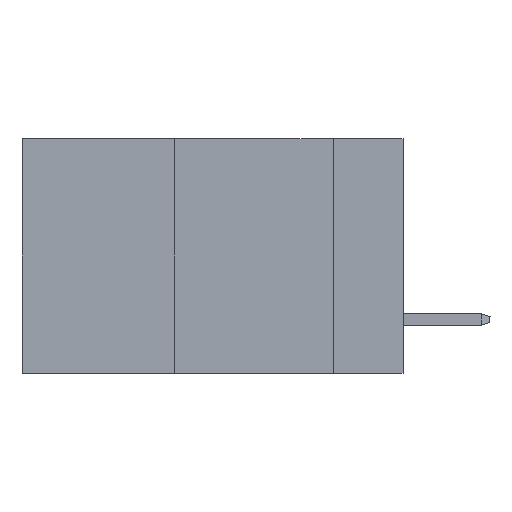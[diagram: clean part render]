
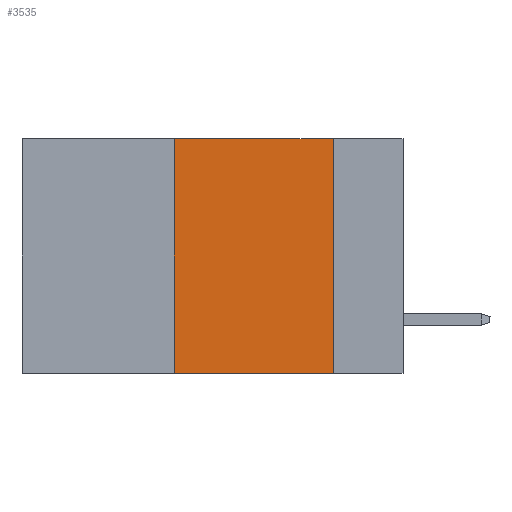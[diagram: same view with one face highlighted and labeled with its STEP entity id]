
A CAD part, left-side view. The second image highlights one B-rep face of the part: STEP entity #3535.
In plain terms, the highlighted planar face has unit normal (-1, 0, 0).
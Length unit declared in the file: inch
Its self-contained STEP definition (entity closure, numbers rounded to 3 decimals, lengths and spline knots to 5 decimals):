
#7 = VERTEX_POINT ( 'NONE', #961 ) ;
#499 = EDGE_CURVE ( 'NONE', #11316, #6173, #6499, .T. ) ;
#673 = VECTOR ( 'NONE', #5587, 39.37008 ) ;
#788 = VERTEX_POINT ( 'NONE', #6085 ) ;
#887 = CARTESIAN_POINT ( 'NONE',  ( 0., 0.6, 0. ) ) ;
#961 = CARTESIAN_POINT ( 'NONE',  ( 0., 0.11, -0.37 ) ) ;
#1082 = CARTESIAN_POINT ( 'NONE',  ( 0., 0.36, -0.37 ) ) ;
#1715 = LINE ( 'NONE', #9124, #1808 ) ;
#1808 = VECTOR ( 'NONE', #6404, 39.37008 ) ;
#2622 = LINE ( 'NONE', #6333, #10935 ) ;
#2680 = VECTOR ( 'NONE', #7737, 39.37008 ) ;
#3228 = DIRECTION ( 'NONE',  ( 0., 0., -1. ) ) ;
#3288 = FACE_OUTER_BOUND ( 'NONE', #8547, .T. ) ;
#3327 = EDGE_CURVE ( 'NONE', #6173, #788, #5530, .T. ) ;
#3535 = ADVANCED_FACE ( 'NONE', ( #3288 ), #5230, .F. ) ;
#3984 = ORIENTED_EDGE ( 'NONE', *, *, #10456, .F. ) ;
#4071 = AXIS2_PLACEMENT_3D ( 'NONE', #6933, #11577, #3228 ) ;
#4265 = ORIENTED_EDGE ( 'NONE', *, *, #9320, .T. ) ;
#5230 = PLANE ( 'NONE',  #4071 ) ;
#5530 = LINE ( 'NONE', #887, #2680 ) ;
#5541 = DIRECTION ( 'NONE',  ( 0., -1., 0. ) ) ;
#5587 = DIRECTION ( 'NONE',  ( 0., 0., 1. ) ) ;
#6085 = CARTESIAN_POINT ( 'NONE',  ( 0., 0.11, 0. ) ) ;
#6173 = VERTEX_POINT ( 'NONE', #10895 ) ;
#6333 = CARTESIAN_POINT ( 'NONE',  ( 0., 0.6, -0.37 ) ) ;
#6404 = DIRECTION ( 'NONE',  ( 0., 0., -1. ) ) ;
#6499 = LINE ( 'NONE', #10199, #673 ) ;
#6933 = CARTESIAN_POINT ( 'NONE',  ( 0., 0.6, 0. ) ) ;
#7737 = DIRECTION ( 'NONE',  ( 0., -1., 0. ) ) ;
#8547 = EDGE_LOOP ( 'NONE', ( #3984, #9746, #10998, #4265 ) ) ;
#9124 = CARTESIAN_POINT ( 'NONE',  ( 0., 0.11, 0. ) ) ;
#9320 = EDGE_CURVE ( 'NONE', #11316, #7, #2622, .T. ) ;
#9746 = ORIENTED_EDGE ( 'NONE', *, *, #3327, .F. ) ;
#10199 = CARTESIAN_POINT ( 'NONE',  ( 0., 0.36, 0. ) ) ;
#10456 = EDGE_CURVE ( 'NONE', #788, #7, #1715, .T. ) ;
#10895 = CARTESIAN_POINT ( 'NONE',  ( 0., 0.36, 0. ) ) ;
#10935 = VECTOR ( 'NONE', #5541, 39.37008 ) ;
#10998 = ORIENTED_EDGE ( 'NONE', *, *, #499, .F. ) ;
#11316 = VERTEX_POINT ( 'NONE', #1082 ) ;
#11577 = DIRECTION ( 'NONE',  ( 1., 0., 0. ) ) ;
